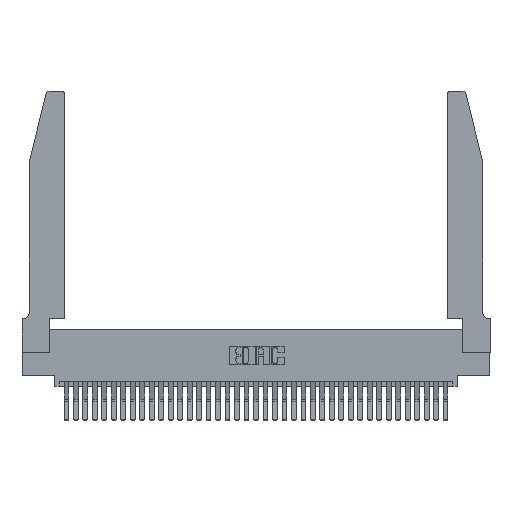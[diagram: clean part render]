
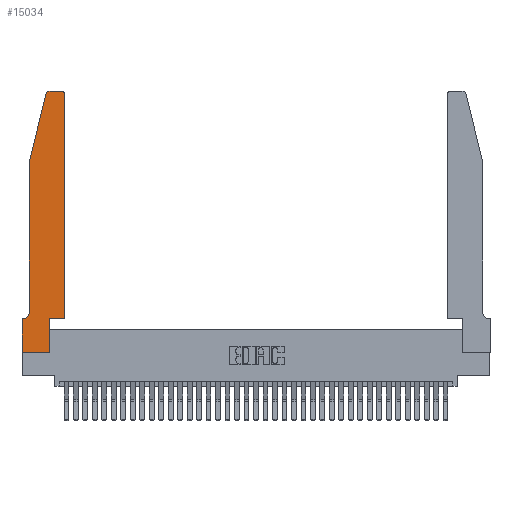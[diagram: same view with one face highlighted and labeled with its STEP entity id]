
A CAD part, top view. The second image highlights one B-rep face of the part: STEP entity #15034.
In plain terms, the highlighted planar face has unit normal (0, 0, 1).
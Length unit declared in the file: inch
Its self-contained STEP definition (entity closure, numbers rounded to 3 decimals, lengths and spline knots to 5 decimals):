
#33 = EDGE_CURVE ( 'NONE', #13208, #5968, #22943, .T. ) ;
#291 = EDGE_LOOP ( 'NONE', ( #4251, #19675, #6061, #13817, #36580, #31725, #11551, #26823, #12442, #21934, #7429, #17007 ) ) ;
#777 = VERTEX_POINT ( 'NONE', #31586 ) ;
#1123 = CARTESIAN_POINT ( 'NONE',  ( 0.4205, 2.72, 0.37 ) ) ;
#1205 = CARTESIAN_POINT ( 'NONE',  ( 0.284, 2.75, 0.37 ) ) ;
#1396 = VERTEX_POINT ( 'NONE', #28812 ) ;
#1471 = DIRECTION ( 'NONE',  ( -1., 0., 0. ) ) ;
#1798 = DIRECTION ( 'NONE',  ( 0., -1., 0. ) ) ;
#1857 = DIRECTION ( 'NONE',  ( -1., 0., 0. ) ) ;
#2175 = EDGE_CURVE ( 'NONE', #4942, #21579, #16090, .T. ) ;
#2257 = AXIS2_PLACEMENT_3D ( 'NONE', #35921, #18869, #1471 ) ;
#2356 = VERTEX_POINT ( 'NONE', #1205 ) ;
#2750 = FACE_OUTER_BOUND ( 'NONE', #291, .T. ) ;
#3288 = LINE ( 'NONE', #6921, #32969 ) ;
#3300 = DIRECTION ( 'NONE',  ( 0., 1., 0. ) ) ;
#3657 = VERTEX_POINT ( 'NONE', #14103 ) ;
#3751 = AXIS2_PLACEMENT_3D ( 'NONE', #31935, #14799, #34764 ) ;
#4092 = DIRECTION ( 'NONE',  ( 1., 0., 0. ) ) ;
#4251 = ORIENTED_EDGE ( 'NONE', *, *, #24771, .T. ) ;
#4942 = VERTEX_POINT ( 'NONE', #34614 ) ;
#5355 = VECTOR ( 'NONE', #1798, 39.37008 ) ;
#5743 = EDGE_CURVE ( 'NONE', #2356, #15257, #19654, .T. ) ;
#5968 = VERTEX_POINT ( 'NONE', #8952 ) ;
#6061 = ORIENTED_EDGE ( 'NONE', *, *, #13657, .T. ) ;
#6203 = EDGE_CURVE ( 'NONE', #31947, #4942, #3288, .T. ) ;
#6322 = EDGE_CURVE ( 'NONE', #1396, #777, #21841, .T. ) ;
#6389 = VERTEX_POINT ( 'NONE', #28099 ) ;
#6428 = VECTOR ( 'NONE', #1857, 39.37008 ) ;
#6570 = VERTEX_POINT ( 'NONE', #34415 ) ;
#6921 = CARTESIAN_POINT ( 'NONE',  ( 0., 0., 0.37 ) ) ;
#7429 = ORIENTED_EDGE ( 'NONE', *, *, #23060, .T. ) ;
#8670 = LINE ( 'NONE', #18720, #15493 ) ;
#8921 = PLANE ( 'NONE',  #3751 ) ;
#8952 = CARTESIAN_POINT ( 'NONE',  ( 0.0755, 0.42, 0.37 ) ) ;
#9459 = CARTESIAN_POINT ( 'NONE',  ( 0.4505, 0.35, 0.37 ) ) ;
#10088 = CARTESIAN_POINT ( 'NONE',  ( 0., 0., 0.37 ) ) ;
#10928 = CARTESIAN_POINT ( 'NONE',  ( 0.0755, 2., 0.37 ) ) ;
#10939 = CARTESIAN_POINT ( 'NONE',  ( 0.284, 2.72, 0.37 ) ) ;
#11551 = ORIENTED_EDGE ( 'NONE', *, *, #32673, .T. ) ;
#11698 = CARTESIAN_POINT ( 'NONE',  ( 0.2605, 2.75, 0.37 ) ) ;
#12442 = ORIENTED_EDGE ( 'NONE', *, *, #2175, .T. ) ;
#12948 = DIRECTION ( 'NONE',  ( 0., 1., 0. ) ) ;
#13153 = VECTOR ( 'NONE', #12948, 39.37008 ) ;
#13208 = VERTEX_POINT ( 'NONE', #10928 ) ;
#13262 = LINE ( 'NONE', #9459, #36046 ) ;
#13476 = EDGE_CURVE ( 'NONE', #21579, #3657, #13262, .T. ) ;
#13657 = EDGE_CURVE ( 'NONE', #15257, #13208, #8670, .T. ) ;
#13817 = ORIENTED_EDGE ( 'NONE', *, *, #33, .T. ) ;
#13860 = DIRECTION ( 'NONE',  ( 1., 0., 0. ) ) ;
#14103 = CARTESIAN_POINT ( 'NONE',  ( 0.4505, 0.35, 0.37 ) ) ;
#14799 = DIRECTION ( 'NONE',  ( 0., 0., 1. ) ) ;
#15034 = ADVANCED_FACE ( 'NONE', ( #2750 ), #8921, .T. ) ;
#15257 = VERTEX_POINT ( 'NONE', #35616 ) ;
#15493 = VECTOR ( 'NONE', #27344, 39.37008 ) ;
#16090 = LINE ( 'NONE', #20635, #17897 ) ;
#16504 = AXIS2_PLACEMENT_3D ( 'NONE', #1123, #21411, #4092 ) ;
#16574 = CIRCLE ( 'NONE', #2257, 0.07 ) ;
#17007 = ORIENTED_EDGE ( 'NONE', *, *, #35575, .T. ) ;
#17897 = VECTOR ( 'NONE', #3300, 39.37008 ) ;
#18720 = CARTESIAN_POINT ( 'NONE',  ( 0.0755, 2., 0.37 ) ) ;
#18844 = LINE ( 'NONE', #11698, #19758 ) ;
#18869 = DIRECTION ( 'NONE',  ( 0., 0., -1. ) ) ;
#19176 = CARTESIAN_POINT ( 'NONE',  ( 0., 0., 0.37 ) ) ;
#19654 = CIRCLE ( 'NONE', #27217, 0.03 ) ;
#19675 = ORIENTED_EDGE ( 'NONE', *, *, #5743, .T. ) ;
#19758 = VECTOR ( 'NONE', #31747, 39.37008 ) ;
#20635 = CARTESIAN_POINT ( 'NONE',  ( 0.2865, 0.35, 0.37 ) ) ;
#20736 = LINE ( 'NONE', #19176, #5355 ) ;
#21411 = DIRECTION ( 'NONE',  ( 0., 0., 1. ) ) ;
#21459 = CIRCLE ( 'NONE', #16504, 0.03 ) ;
#21579 = VERTEX_POINT ( 'NONE', #28703 ) ;
#21841 = LINE ( 'NONE', #27724, #6428 ) ;
#21934 = ORIENTED_EDGE ( 'NONE', *, *, #13476, .T. ) ;
#22409 = CARTESIAN_POINT ( 'NONE',  ( 0.0755, 2., 0.37 ) ) ;
#22943 = LINE ( 'NONE', #22409, #29610 ) ;
#23060 = EDGE_CURVE ( 'NONE', #3657, #6389, #29290, .T. ) ;
#24771 = EDGE_CURVE ( 'NONE', #6570, #2356, #18844, .T. ) ;
#25097 = EDGE_CURVE ( 'NONE', #5968, #1396, #16574, .T. ) ;
#26823 = ORIENTED_EDGE ( 'NONE', *, *, #6203, .T. ) ;
#27217 = AXIS2_PLACEMENT_3D ( 'NONE', #10939, #31013, #13860 ) ;
#27250 = CARTESIAN_POINT ( 'NONE',  ( 0.4505, 0.35, 0.37 ) ) ;
#27344 = DIRECTION ( 'NONE',  ( -0.239, -0.971, 0. ) ) ;
#27724 = CARTESIAN_POINT ( 'NONE',  ( 0.0755, 0.35, 0.37 ) ) ;
#28099 = CARTESIAN_POINT ( 'NONE',  ( 0.4505, 2.72, 0.37 ) ) ;
#28703 = CARTESIAN_POINT ( 'NONE',  ( 0.2865, 0.35, 0.37 ) ) ;
#28812 = CARTESIAN_POINT ( 'NONE',  ( 0.0055, 0.35, 0.37 ) ) ;
#29290 = LINE ( 'NONE', #27250, #13153 ) ;
#29579 = DIRECTION ( 'NONE',  ( 1., 0., 0. ) ) ;
#29610 = VECTOR ( 'NONE', #36802, 39.37008 ) ;
#31013 = DIRECTION ( 'NONE',  ( 0., 0., 1. ) ) ;
#31586 = CARTESIAN_POINT ( 'NONE',  ( 0., 0.35, 0.37 ) ) ;
#31725 = ORIENTED_EDGE ( 'NONE', *, *, #6322, .T. ) ;
#31747 = DIRECTION ( 'NONE',  ( -1., 0., 0. ) ) ;
#31935 = CARTESIAN_POINT ( 'NONE',  ( 0., 0.35, 0.37 ) ) ;
#31947 = VERTEX_POINT ( 'NONE', #10088 ) ;
#32673 = EDGE_CURVE ( 'NONE', #777, #31947, #20736, .T. ) ;
#32969 = VECTOR ( 'NONE', #35648, 39.37008 ) ;
#34415 = CARTESIAN_POINT ( 'NONE',  ( 0.4205, 2.75, 0.37 ) ) ;
#34614 = CARTESIAN_POINT ( 'NONE',  ( 0.2865, 0., 0.37 ) ) ;
#34764 = DIRECTION ( 'NONE',  ( 1., 0., 0. ) ) ;
#35575 = EDGE_CURVE ( 'NONE', #6389, #6570, #21459, .T. ) ;
#35616 = CARTESIAN_POINT ( 'NONE',  ( 0.25487, 2.72718, 0.37 ) ) ;
#35648 = DIRECTION ( 'NONE',  ( 1., 0., 0. ) ) ;
#35921 = CARTESIAN_POINT ( 'NONE',  ( 0.0055, 0.42, 0.37 ) ) ;
#36046 = VECTOR ( 'NONE', #29579, 39.37008 ) ;
#36580 = ORIENTED_EDGE ( 'NONE', *, *, #25097, .T. ) ;
#36802 = DIRECTION ( 'NONE',  ( 0., -1., 0. ) ) ;
